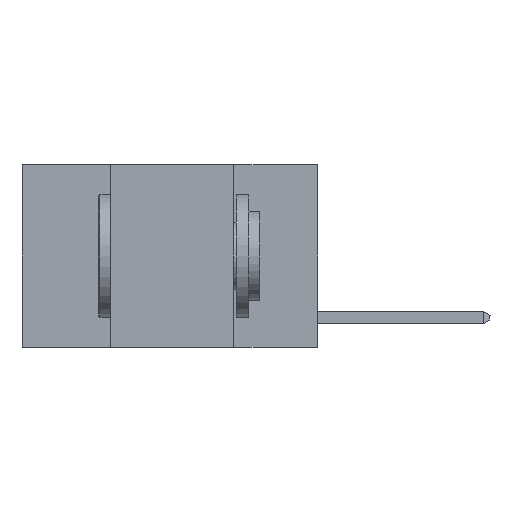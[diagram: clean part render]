
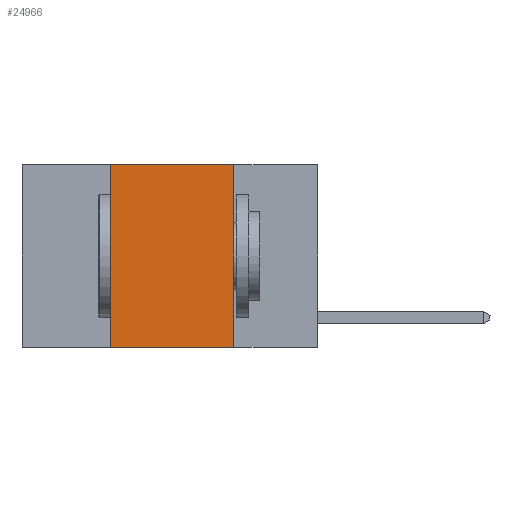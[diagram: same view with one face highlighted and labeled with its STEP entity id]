
A CAD part, left-side view. The second image highlights one B-rep face of the part: STEP entity #24966.
In plain terms, the highlighted planar face has unit normal (-1, 0, 0).
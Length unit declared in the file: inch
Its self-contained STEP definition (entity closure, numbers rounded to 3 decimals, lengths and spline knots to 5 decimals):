
#1704 = VECTOR ( 'NONE', #10898, 39.37008 ) ;
#2428 = VERTEX_POINT ( 'NONE', #5044 ) ;
#2587 = VERTEX_POINT ( 'NONE', #11706 ) ;
#4490 = EDGE_LOOP ( 'NONE', ( #21323, #4740, #18544, #9995 ) ) ;
#4532 = VECTOR ( 'NONE', #6788, 39.37008 ) ;
#4740 = ORIENTED_EDGE ( 'NONE', *, *, #6963, .F. ) ;
#4913 = CARTESIAN_POINT ( 'NONE',  ( 0., 0.42, 0. ) ) ;
#5044 = CARTESIAN_POINT ( 'NONE',  ( 0., 0.42, 0. ) ) ;
#5760 = CARTESIAN_POINT ( 'NONE',  ( 0., 0.17, -0.37 ) ) ;
#6788 = DIRECTION ( 'NONE',  ( 0., 0., -1. ) ) ;
#6963 = EDGE_CURVE ( 'NONE', #2428, #7042, #18459, .T. ) ;
#7042 = VERTEX_POINT ( 'NONE', #11151 ) ;
#7264 = CARTESIAN_POINT ( 'NONE',  ( 0., 0.6, 0. ) ) ;
#7396 = PLANE ( 'NONE',  #19188 ) ;
#9995 = ORIENTED_EDGE ( 'NONE', *, *, #26093, .T. ) ;
#10898 = DIRECTION ( 'NONE',  ( 0., -1., 0. ) ) ;
#11151 = CARTESIAN_POINT ( 'NONE',  ( 0., 0.17, 0. ) ) ;
#11427 = DIRECTION ( 'NONE',  ( 0., 0., -1. ) ) ;
#11706 = CARTESIAN_POINT ( 'NONE',  ( 0., 0.42, -0.37 ) ) ;
#12811 = CARTESIAN_POINT ( 'NONE',  ( 0., 0.17, 0. ) ) ;
#14750 = EDGE_CURVE ( 'NONE', #2587, #2428, #15315, .T. ) ;
#14829 = LINE ( 'NONE', #12811, #4532 ) ;
#15315 = LINE ( 'NONE', #4913, #15513 ) ;
#15416 = DIRECTION ( 'NONE',  ( 1., 0., 0. ) ) ;
#15513 = VECTOR ( 'NONE', #25284, 39.37008 ) ;
#16210 = VERTEX_POINT ( 'NONE', #5760 ) ;
#16258 = LINE ( 'NONE', #24404, #1704 ) ;
#18459 = LINE ( 'NONE', #22620, #22401 ) ;
#18544 = ORIENTED_EDGE ( 'NONE', *, *, #14750, .F. ) ;
#19188 = AXIS2_PLACEMENT_3D ( 'NONE', #7264, #15416, #11427 ) ;
#19969 = EDGE_CURVE ( 'NONE', #7042, #16210, #14829, .T. ) ;
#21323 = ORIENTED_EDGE ( 'NONE', *, *, #19969, .F. ) ;
#22401 = VECTOR ( 'NONE', #25106, 39.37008 ) ;
#22620 = CARTESIAN_POINT ( 'NONE',  ( 0., 0.6, 0. ) ) ;
#24404 = CARTESIAN_POINT ( 'NONE',  ( 0., 0.6, -0.37 ) ) ;
#24966 = ADVANCED_FACE ( 'NONE', ( #25521 ), #7396, .F. ) ;
#25106 = DIRECTION ( 'NONE',  ( 0., -1., 0. ) ) ;
#25284 = DIRECTION ( 'NONE',  ( 0., 0., 1. ) ) ;
#25521 = FACE_OUTER_BOUND ( 'NONE', #4490, .T. ) ;
#26093 = EDGE_CURVE ( 'NONE', #2587, #16210, #16258, .T. ) ;
